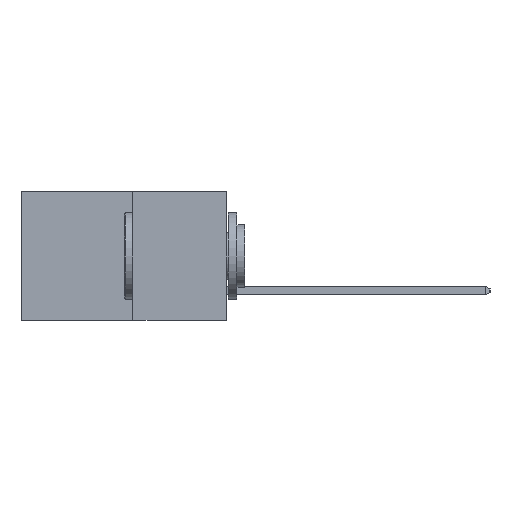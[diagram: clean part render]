
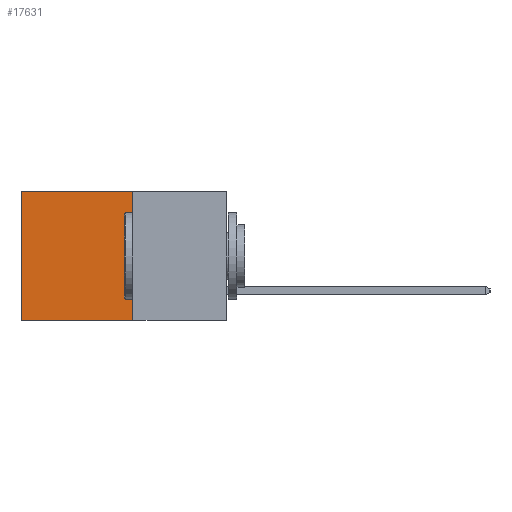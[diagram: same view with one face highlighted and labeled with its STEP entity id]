
A CAD part, left-side view. The second image highlights one B-rep face of the part: STEP entity #17631.
In plain terms, the highlighted planar face has unit normal (-1, 0, 0).
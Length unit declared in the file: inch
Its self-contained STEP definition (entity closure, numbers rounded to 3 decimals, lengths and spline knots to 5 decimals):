
#1045 = CARTESIAN_POINT ( 'NONE',  ( 0.277, 0.27, -0.37 ) ) ;
#2921 = DIRECTION ( 'NONE',  ( 0., 0., -1. ) ) ;
#3635 = EDGE_CURVE ( 'NONE', #23256, #10609, #12271, .T. ) ;
#3668 = DIRECTION ( 'NONE',  ( 1., 0., 0. ) ) ;
#4866 = VECTOR ( 'NONE', #2921, 39.37008 ) ;
#5815 = LINE ( 'NONE', #16161, #31302 ) ;
#8098 = VERTEX_POINT ( 'NONE', #23855 ) ;
#8754 = EDGE_CURVE ( 'NONE', #23256, #8098, #10307, .T. ) ;
#9194 = CARTESIAN_POINT ( 'NONE',  ( 0.277, 0.59, -0.37 ) ) ;
#9620 = EDGE_CURVE ( 'NONE', #10609, #27498, #12745, .T. ) ;
#10307 = LINE ( 'NONE', #18777, #4866 ) ;
#10403 = CARTESIAN_POINT ( 'NONE',  ( 0.277, 0.59, 0. ) ) ;
#10609 = VERTEX_POINT ( 'NONE', #10403 ) ;
#11853 = DIRECTION ( 'NONE',  ( 0., 0., -1. ) ) ;
#12271 = LINE ( 'NONE', #30271, #13963 ) ;
#12745 = LINE ( 'NONE', #9194, #31920 ) ;
#13404 = CARTESIAN_POINT ( 'NONE',  ( 0.277, 0.59, -0.37 ) ) ;
#13963 = VECTOR ( 'NONE', #30146, 39.37008 ) ;
#14349 = EDGE_CURVE ( 'NONE', #8098, #27498, #5815, .T. ) ;
#16161 = CARTESIAN_POINT ( 'NONE',  ( 0.277, 0.27, -0.37 ) ) ;
#17631 = ADVANCED_FACE ( 'NONE', ( #22561 ), #32472, .F. ) ;
#18755 = DIRECTION ( 'NONE',  ( 0., 1., 0. ) ) ;
#18777 = CARTESIAN_POINT ( 'NONE',  ( 0.277, 0.27, -0.37 ) ) ;
#18791 = EDGE_LOOP ( 'NONE', ( #26135, #27220, #23811, #19004 ) ) ;
#19004 = ORIENTED_EDGE ( 'NONE', *, *, #3635, .T. ) ;
#22127 = DIRECTION ( 'NONE',  ( 0., 0., -1. ) ) ;
#22561 = FACE_OUTER_BOUND ( 'NONE', #18791, .T. ) ;
#23256 = VERTEX_POINT ( 'NONE', #25052 ) ;
#23811 = ORIENTED_EDGE ( 'NONE', *, *, #8754, .F. ) ;
#23855 = CARTESIAN_POINT ( 'NONE',  ( 0.277, 0.27, -0.37 ) ) ;
#25052 = CARTESIAN_POINT ( 'NONE',  ( 0.277, 0.27, 0. ) ) ;
#26135 = ORIENTED_EDGE ( 'NONE', *, *, #9620, .T. ) ;
#27220 = ORIENTED_EDGE ( 'NONE', *, *, #14349, .F. ) ;
#27498 = VERTEX_POINT ( 'NONE', #13404 ) ;
#30144 = AXIS2_PLACEMENT_3D ( 'NONE', #1045, #3668, #22127 ) ;
#30146 = DIRECTION ( 'NONE',  ( 0., 1., 0. ) ) ;
#30271 = CARTESIAN_POINT ( 'NONE',  ( 0.277, 0.27, 0. ) ) ;
#31302 = VECTOR ( 'NONE', #18755, 39.37008 ) ;
#31920 = VECTOR ( 'NONE', #11853, 39.37008 ) ;
#32472 = PLANE ( 'NONE',  #30144 ) ;
